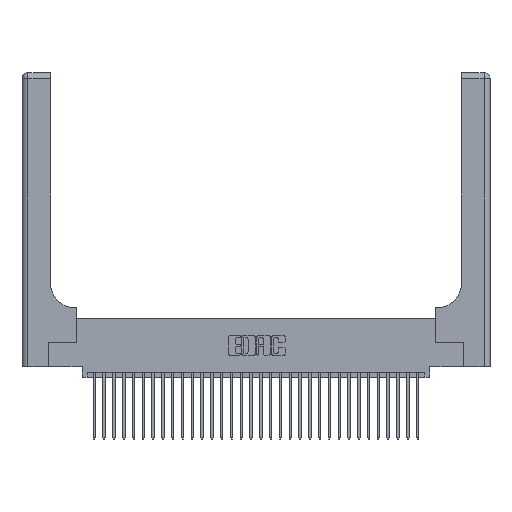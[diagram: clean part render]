
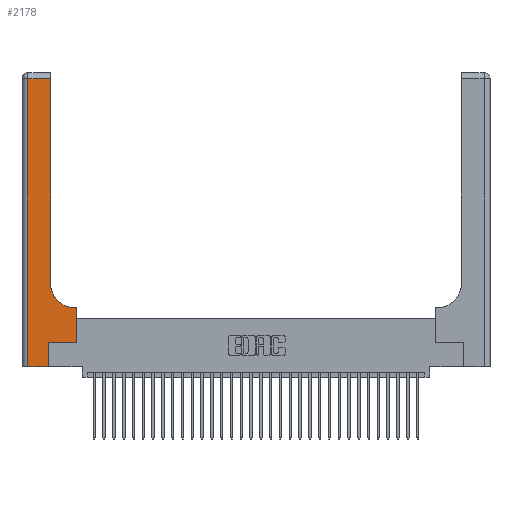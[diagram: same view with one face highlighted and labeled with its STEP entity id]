
A CAD part, top view. The second image highlights one B-rep face of the part: STEP entity #2178.
In plain terms, the highlighted planar face has unit normal (0, 0, 1).
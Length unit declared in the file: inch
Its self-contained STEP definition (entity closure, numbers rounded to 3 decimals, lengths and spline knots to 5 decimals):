
#795 = CARTESIAN_POINT ( 'NONE',  ( 0.06, 3., 0.37 ) ) ;
#944 = VERTEX_POINT ( 'NONE', #20569 ) ;
#973 = CARTESIAN_POINT ( 'NONE',  ( 0.06, 0., 0.37 ) ) ;
#1565 = VECTOR ( 'NONE', #13537, 39.37008 ) ;
#2178 = ADVANCED_FACE ( 'NONE', ( #4843 ), #17616, .F. ) ;
#2292 = CARTESIAN_POINT ( 'NONE',  ( 0., 3., 0.37 ) ) ;
#2715 = DIRECTION ( 'NONE',  ( 0., 0., -1. ) ) ;
#3581 = VERTEX_POINT ( 'NONE', #16932 ) ;
#3662 = CARTESIAN_POINT ( 'NONE',  ( 0.269, 0.25, 0.37 ) ) ;
#4825 = EDGE_CURVE ( 'NONE', #20707, #31806, #20639, .T. ) ;
#4843 = FACE_OUTER_BOUND ( 'NONE', #22849, .T. ) ;
#4866 = VECTOR ( 'NONE', #6538, 39.37008 ) ;
#6329 = ORIENTED_EDGE ( 'NONE', *, *, #11292, .T. ) ;
#6396 = DIRECTION ( 'NONE',  ( -1., 0., 0. ) ) ;
#6538 = DIRECTION ( 'NONE',  ( 0., 1., 0. ) ) ;
#6771 = VERTEX_POINT ( 'NONE', #21844 ) ;
#6804 = LINE ( 'NONE', #7519, #1565 ) ;
#7303 = DIRECTION ( 'NONE',  ( 1., 0., 0. ) ) ;
#7426 = EDGE_CURVE ( 'NONE', #8881, #944, #6804, .T. ) ;
#7446 = DIRECTION ( 'NONE',  ( -1., 0., 0. ) ) ;
#7519 = CARTESIAN_POINT ( 'NONE',  ( 0., 0., 0.37 ) ) ;
#7602 = VERTEX_POINT ( 'NONE', #19221 ) ;
#7813 = VECTOR ( 'NONE', #7303, 39.37008 ) ;
#8648 = CARTESIAN_POINT ( 'NONE',  ( 0.5415, 0.6, 0.37 ) ) ;
#8848 = LINE ( 'NONE', #32082, #12435 ) ;
#8881 = VERTEX_POINT ( 'NONE', #973 ) ;
#10720 = CARTESIAN_POINT ( 'NONE',  ( 0.2915, 0.85, 0.37 ) ) ;
#11292 = EDGE_CURVE ( 'NONE', #22165, #3581, #28848, .T. ) ;
#11925 = EDGE_CURVE ( 'NONE', #7602, #20707, #8848, .T. ) ;
#12435 = VECTOR ( 'NONE', #6396, 39.37008 ) ;
#12570 = DIRECTION ( 'NONE',  ( 1., 0., 0. ) ) ;
#13537 = DIRECTION ( 'NONE',  ( 1., 0., 0. ) ) ;
#13862 = LINE ( 'NONE', #22604, #7813 ) ;
#14086 = ORIENTED_EDGE ( 'NONE', *, *, #32655, .T. ) ;
#15150 = DIRECTION ( 'NONE',  ( -1., 0., 0. ) ) ;
#16792 = CARTESIAN_POINT ( 'NONE',  ( 0.269, 0., 0.37 ) ) ;
#16886 = LINE ( 'NONE', #19160, #4866 ) ;
#16894 = DIRECTION ( 'NONE',  ( 0., 1., 0. ) ) ;
#16932 = CARTESIAN_POINT ( 'NONE',  ( 0.06, 2.94, 0.37 ) ) ;
#16965 = DIRECTION ( 'NONE',  ( 0., 0., -1. ) ) ;
#17616 = PLANE ( 'NONE',  #23187 ) ;
#17789 = VECTOR ( 'NONE', #32127, 39.37008 ) ;
#18192 = VERTEX_POINT ( 'NONE', #3662 ) ;
#18321 = EDGE_CURVE ( 'NONE', #6771, #7602, #19506, .T. ) ;
#19160 = CARTESIAN_POINT ( 'NONE',  ( 0.2915, 3., 0.37 ) ) ;
#19206 = DIRECTION ( 'NONE',  ( 0., 1., 0. ) ) ;
#19221 = CARTESIAN_POINT ( 'NONE',  ( 0.5585, 0.6, 0.37 ) ) ;
#19506 = LINE ( 'NONE', #24090, #26247 ) ;
#19690 = VECTOR ( 'NONE', #15150, 39.37008 ) ;
#19983 = CARTESIAN_POINT ( 'NONE',  ( 0.2915, 2.94, 0.37 ) ) ;
#20320 = EDGE_CURVE ( 'NONE', #18192, #6771, #13862, .T. ) ;
#20569 = CARTESIAN_POINT ( 'NONE',  ( 0.269, 0., 0.37 ) ) ;
#20639 = CIRCLE ( 'NONE', #26000, 0.25 ) ;
#20707 = VERTEX_POINT ( 'NONE', #8648 ) ;
#20973 = LINE ( 'NONE', #795, #17789 ) ;
#21473 = ORIENTED_EDGE ( 'NONE', *, *, #4825, .T. ) ;
#21844 = CARTESIAN_POINT ( 'NONE',  ( 0.5585, 0.25, 0.37 ) ) ;
#22165 = VERTEX_POINT ( 'NONE', #19983 ) ;
#22604 = CARTESIAN_POINT ( 'NONE',  ( 0.269, 0.25, 0.37 ) ) ;
#22849 = EDGE_LOOP ( 'NONE', ( #22869, #6329, #14086, #23772, #28888, #27464, #25799, #31861, #21473 ) ) ;
#22869 = ORIENTED_EDGE ( 'NONE', *, *, #28390, .T. ) ;
#23187 = AXIS2_PLACEMENT_3D ( 'NONE', #2292, #2715, #7446 ) ;
#23772 = ORIENTED_EDGE ( 'NONE', *, *, #7426, .T. ) ;
#24090 = CARTESIAN_POINT ( 'NONE',  ( 0.5585, 0.25, 0.37 ) ) ;
#24696 = LINE ( 'NONE', #16792, #26277 ) ;
#25063 = CARTESIAN_POINT ( 'NONE',  ( 0.5415, 0.85, 0.37 ) ) ;
#25265 = CARTESIAN_POINT ( 'NONE',  ( 0., 2.94, 0.37 ) ) ;
#25799 = ORIENTED_EDGE ( 'NONE', *, *, #18321, .T. ) ;
#26000 = AXIS2_PLACEMENT_3D ( 'NONE', #25063, #16965, #12570 ) ;
#26247 = VECTOR ( 'NONE', #19206, 39.37008 ) ;
#26277 = VECTOR ( 'NONE', #16894, 39.37008 ) ;
#27464 = ORIENTED_EDGE ( 'NONE', *, *, #20320, .T. ) ;
#28390 = EDGE_CURVE ( 'NONE', #31806, #22165, #16886, .T. ) ;
#28848 = LINE ( 'NONE', #25265, #19690 ) ;
#28888 = ORIENTED_EDGE ( 'NONE', *, *, #30286, .T. ) ;
#30286 = EDGE_CURVE ( 'NONE', #944, #18192, #24696, .T. ) ;
#31806 = VERTEX_POINT ( 'NONE', #10720 ) ;
#31861 = ORIENTED_EDGE ( 'NONE', *, *, #11925, .T. ) ;
#32082 = CARTESIAN_POINT ( 'NONE',  ( 0.2915, 0.6, 0.37 ) ) ;
#32127 = DIRECTION ( 'NONE',  ( 0., -1., 0. ) ) ;
#32655 = EDGE_CURVE ( 'NONE', #3581, #8881, #20973, .T. ) ;
